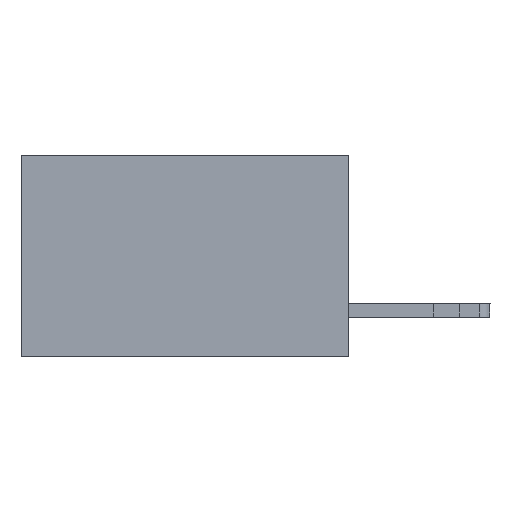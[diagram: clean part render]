
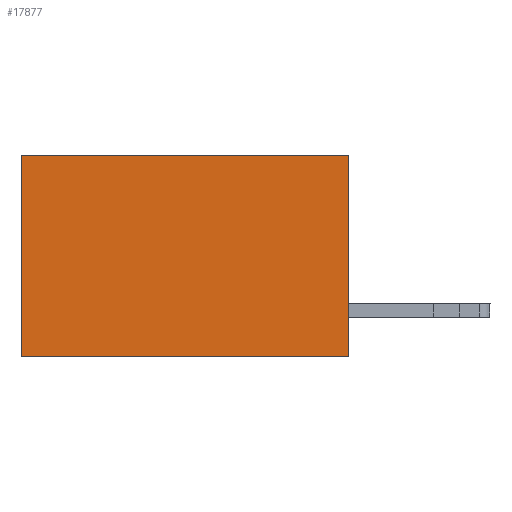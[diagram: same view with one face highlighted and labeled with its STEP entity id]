
A CAD part, left-side view. The second image highlights one B-rep face of the part: STEP entity #17877.
In plain terms, the highlighted planar face has unit normal (-1, 0, 0).
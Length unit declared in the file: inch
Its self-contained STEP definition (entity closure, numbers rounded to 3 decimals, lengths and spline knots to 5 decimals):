
#813 = CARTESIAN_POINT ( 'NONE',  ( 0.2615, 0.6, -0.37 ) ) ;
#1027 = CARTESIAN_POINT ( 'NONE',  ( 0.2615, 0., 0. ) ) ;
#1130 = AXIS2_PLACEMENT_3D ( 'NONE', #10301, #7342, #2682 ) ;
#1505 = ORIENTED_EDGE ( 'NONE', *, *, #18526, .T. ) ;
#1677 = LINE ( 'NONE', #14878, #12777 ) ;
#2682 = DIRECTION ( 'NONE',  ( 0., 0., -1. ) ) ;
#3864 = EDGE_CURVE ( 'NONE', #7786, #15577, #17181, .T. ) ;
#4403 = VECTOR ( 'NONE', #14541, 39.37008 ) ;
#4591 = EDGE_CURVE ( 'NONE', #7683, #7786, #1677, .T. ) ;
#5897 = LINE ( 'NONE', #813, #13241 ) ;
#5946 = VERTEX_POINT ( 'NONE', #9186 ) ;
#7342 = DIRECTION ( 'NONE',  ( 1., 0., 0. ) ) ;
#7683 = VERTEX_POINT ( 'NONE', #11001 ) ;
#7786 = VERTEX_POINT ( 'NONE', #8139 ) ;
#8139 = CARTESIAN_POINT ( 'NONE',  ( 0.2615, 0., -0.37 ) ) ;
#8220 = EDGE_LOOP ( 'NONE', ( #1505, #18177, #11536, #8432 ) ) ;
#8346 = DIRECTION ( 'NONE',  ( 0., 1., 0. ) ) ;
#8371 = CARTESIAN_POINT ( 'NONE',  ( 0.2615, 0., -0.37 ) ) ;
#8432 = ORIENTED_EDGE ( 'NONE', *, *, #18626, .T. ) ;
#9186 = CARTESIAN_POINT ( 'NONE',  ( 0.2615, 0.6, 0. ) ) ;
#10301 = CARTESIAN_POINT ( 'NONE',  ( 0.2615, 0., -0.37 ) ) ;
#11001 = CARTESIAN_POINT ( 'NONE',  ( 0.2615, 0., 0. ) ) ;
#11536 = ORIENTED_EDGE ( 'NONE', *, *, #4591, .F. ) ;
#11721 = PLANE ( 'NONE',  #1130 ) ;
#11884 = LINE ( 'NONE', #1027, #4403 ) ;
#12777 = VECTOR ( 'NONE', #13408, 39.37008 ) ;
#13241 = VECTOR ( 'NONE', #14422, 39.37008 ) ;
#13408 = DIRECTION ( 'NONE',  ( 0., 0., -1. ) ) ;
#13719 = CARTESIAN_POINT ( 'NONE',  ( 0.2615, 0.6, -0.37 ) ) ;
#13901 = VECTOR ( 'NONE', #8346, 39.37008 ) ;
#14422 = DIRECTION ( 'NONE',  ( 0., 0., -1. ) ) ;
#14541 = DIRECTION ( 'NONE',  ( 0., 1., 0. ) ) ;
#14790 = FACE_OUTER_BOUND ( 'NONE', #8220, .T. ) ;
#14878 = CARTESIAN_POINT ( 'NONE',  ( 0.2615, 0., -0.37 ) ) ;
#15577 = VERTEX_POINT ( 'NONE', #13719 ) ;
#17181 = LINE ( 'NONE', #8371, #13901 ) ;
#17877 = ADVANCED_FACE ( 'NONE', ( #14790 ), #11721, .F. ) ;
#18177 = ORIENTED_EDGE ( 'NONE', *, *, #3864, .F. ) ;
#18526 = EDGE_CURVE ( 'NONE', #5946, #15577, #5897, .T. ) ;
#18626 = EDGE_CURVE ( 'NONE', #7683, #5946, #11884, .T. ) ;
